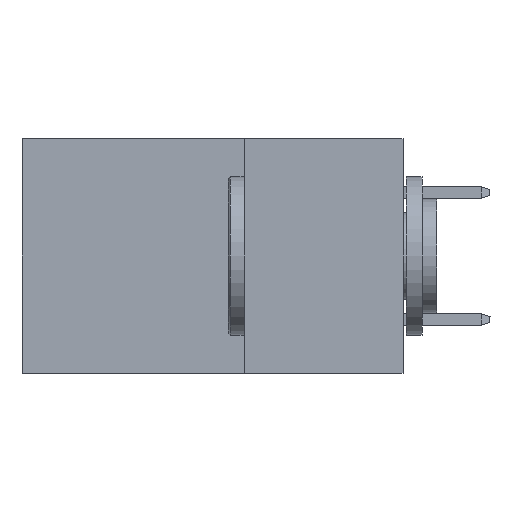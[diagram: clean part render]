
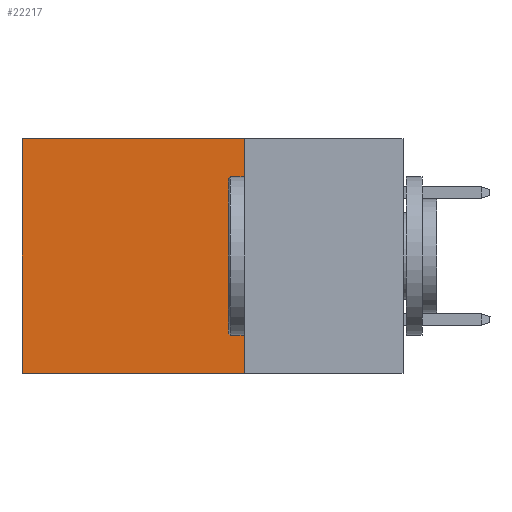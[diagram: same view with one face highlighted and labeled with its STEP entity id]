
A CAD part, left-side view. The second image highlights one B-rep face of the part: STEP entity #22217.
In plain terms, the highlighted planar face has unit normal (-1, 0, 0).
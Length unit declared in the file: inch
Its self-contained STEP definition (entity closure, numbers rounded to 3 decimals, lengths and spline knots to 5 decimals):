
#75 = DIRECTION ( 'NONE',  ( 0., 1., 0. ) ) ;
#801 = VERTEX_POINT ( 'NONE', #13895 ) ;
#1376 = PLANE ( 'NONE',  #18681 ) ;
#1494 = DIRECTION ( 'NONE',  ( 0., 0., -1. ) ) ;
#1791 = CARTESIAN_POINT ( 'NONE',  ( 0.2875, 0.25, 0. ) ) ;
#2868 = DIRECTION ( 'NONE',  ( 0., 0., -1. ) ) ;
#3061 = CARTESIAN_POINT ( 'NONE',  ( 0.2875, 0.25, -0.37 ) ) ;
#5033 = CARTESIAN_POINT ( 'NONE',  ( 0.2875, 0.25, 0. ) ) ;
#6118 = EDGE_CURVE ( 'NONE', #13525, #25947, #6862, .T. ) ;
#6862 = LINE ( 'NONE', #20162, #22844 ) ;
#7757 = VECTOR ( 'NONE', #2868, 39.37008 ) ;
#8264 = EDGE_CURVE ( 'NONE', #25947, #16101, #12451, .T. ) ;
#8749 = VECTOR ( 'NONE', #16213, 39.37008 ) ;
#10089 = VECTOR ( 'NONE', #1494, 39.37008 ) ;
#10162 = DIRECTION ( 'NONE',  ( 0., 0., -1. ) ) ;
#10309 = FACE_OUTER_BOUND ( 'NONE', #20178, .T. ) ;
#12451 = LINE ( 'NONE', #21279, #10089 ) ;
#13525 = VERTEX_POINT ( 'NONE', #21278 ) ;
#13895 = CARTESIAN_POINT ( 'NONE',  ( 0.2875, 0.25, -0.37 ) ) ;
#14061 = LINE ( 'NONE', #3061, #8749 ) ;
#14160 = ORIENTED_EDGE ( 'NONE', *, *, #18291, .F. ) ;
#14176 = EDGE_CURVE ( 'NONE', #13525, #801, #22504, .T. ) ;
#16101 = VERTEX_POINT ( 'NONE', #23336 ) ;
#16213 = DIRECTION ( 'NONE',  ( 0., 1., 0. ) ) ;
#17901 = ORIENTED_EDGE ( 'NONE', *, *, #14176, .F. ) ;
#18291 = EDGE_CURVE ( 'NONE', #801, #16101, #14061, .T. ) ;
#18681 = AXIS2_PLACEMENT_3D ( 'NONE', #1791, #23446, #10162 ) ;
#20162 = CARTESIAN_POINT ( 'NONE',  ( 0.2875, 0.25, 0. ) ) ;
#20178 = EDGE_LOOP ( 'NONE', ( #27627, #14160, #17901, #27093 ) ) ;
#21278 = CARTESIAN_POINT ( 'NONE',  ( 0.2875, 0.25, 0. ) ) ;
#21279 = CARTESIAN_POINT ( 'NONE',  ( 0.2875, 0.6, 0. ) ) ;
#22217 = ADVANCED_FACE ( 'NONE', ( #10309 ), #1376, .F. ) ;
#22504 = LINE ( 'NONE', #5033, #7757 ) ;
#22844 = VECTOR ( 'NONE', #75, 39.37008 ) ;
#23336 = CARTESIAN_POINT ( 'NONE',  ( 0.2875, 0.6, -0.37 ) ) ;
#23446 = DIRECTION ( 'NONE',  ( 1., 0., 0. ) ) ;
#24834 = CARTESIAN_POINT ( 'NONE',  ( 0.2875, 0.6, 0. ) ) ;
#25947 = VERTEX_POINT ( 'NONE', #24834 ) ;
#27093 = ORIENTED_EDGE ( 'NONE', *, *, #6118, .T. ) ;
#27627 = ORIENTED_EDGE ( 'NONE', *, *, #8264, .T. ) ;
